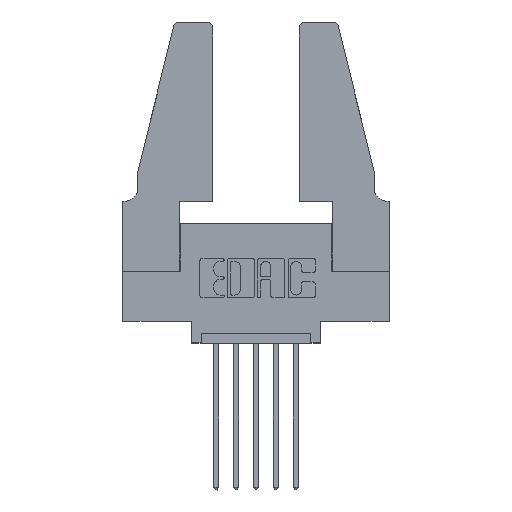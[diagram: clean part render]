
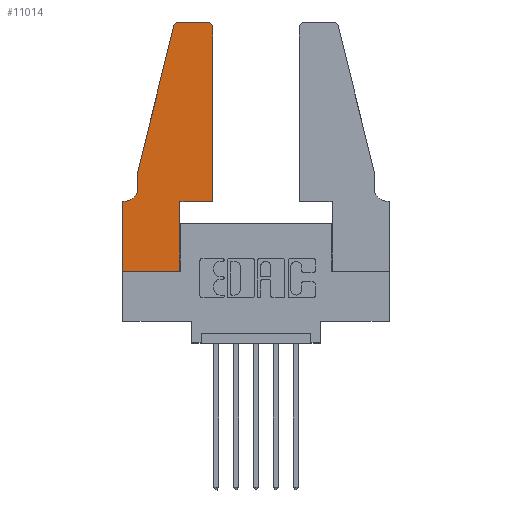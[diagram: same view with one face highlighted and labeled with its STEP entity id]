
A CAD part, top view. The second image highlights one B-rep face of the part: STEP entity #11014.
In plain terms, the highlighted planar face has unit normal (0, 0, 1).
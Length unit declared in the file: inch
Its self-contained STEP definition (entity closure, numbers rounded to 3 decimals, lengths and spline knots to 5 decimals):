
#429 = VERTEX_POINT ( 'NONE', #3707 ) ;
#541 = VECTOR ( 'NONE', #5327, 39.37008 ) ;
#584 = CARTESIAN_POINT ( 'NONE',  ( 0.4205, 1.25, 0.37 ) ) ;
#663 = CARTESIAN_POINT ( 'NONE',  ( 0., 0., 0.37 ) ) ;
#728 = CARTESIAN_POINT ( 'NONE',  ( 0.4505, 0.35, 0.37 ) ) ;
#730 = CIRCLE ( 'NONE', #3010, 0.03 ) ;
#745 = DIRECTION ( 'NONE',  ( -1., 0., 0. ) ) ;
#778 = CARTESIAN_POINT ( 'NONE',  ( 0.2865, 0.35, 0.37 ) ) ;
#1076 = ORIENTED_EDGE ( 'NONE', *, *, #3592, .T. ) ;
#1146 = LINE ( 'NONE', #728, #5699 ) ;
#1365 = DIRECTION ( 'NONE',  ( 1., 0., 0. ) ) ;
#1618 = DIRECTION ( 'NONE',  ( 0., 1., 0. ) ) ;
#1673 = DIRECTION ( 'NONE',  ( 0., 1., 0. ) ) ;
#1690 = CARTESIAN_POINT ( 'NONE',  ( 0.2865, 0., 0.37 ) ) ;
#1817 = VERTEX_POINT ( 'NONE', #10746 ) ;
#1918 = DIRECTION ( 'NONE',  ( -1., 0., 0. ) ) ;
#1926 = AXIS2_PLACEMENT_3D ( 'NONE', #5299, #6277, #3754 ) ;
#1953 = EDGE_CURVE ( 'NONE', #7931, #5678, #6716, .T. ) ;
#2191 = DIRECTION ( 'NONE',  ( -0.239, -0.971, 0. ) ) ;
#2199 = VERTEX_POINT ( 'NONE', #4493 ) ;
#2353 = VECTOR ( 'NONE', #1918, 39.37008 ) ;
#2553 = VECTOR ( 'NONE', #1365, 39.37008 ) ;
#2672 = EDGE_CURVE ( 'NONE', #7817, #1817, #7754, .T. ) ;
#2702 = EDGE_CURVE ( 'NONE', #5678, #7817, #6562, .T. ) ;
#2801 = CARTESIAN_POINT ( 'NONE',  ( 0., 0.35, 0.37 ) ) ;
#2839 = DIRECTION ( 'NONE',  ( 1., 0., 0. ) ) ;
#3010 = AXIS2_PLACEMENT_3D ( 'NONE', #9681, #10557, #8020 ) ;
#3168 = CARTESIAN_POINT ( 'NONE',  ( 0.0755, 0.5, 0.37 ) ) ;
#3229 = EDGE_CURVE ( 'NONE', #5174, #7931, #8313, .T. ) ;
#3278 = EDGE_CURVE ( 'NONE', #8522, #9363, #4676, .T. ) ;
#3303 = ORIENTED_EDGE ( 'NONE', *, *, #2702, .T. ) ;
#3383 = DIRECTION ( 'NONE',  ( 0., 0., -1. ) ) ;
#3541 = ORIENTED_EDGE ( 'NONE', *, *, #10497, .T. ) ;
#3592 = EDGE_CURVE ( 'NONE', #4419, #7984, #6683, .T. ) ;
#3603 = VECTOR ( 'NONE', #8098, 39.37008 ) ;
#3707 = CARTESIAN_POINT ( 'NONE',  ( 0.0755, 0.42, 0.37 ) ) ;
#3754 = DIRECTION ( 'NONE',  ( 1., 0., 0. ) ) ;
#3894 = DIRECTION ( 'NONE',  ( -1., 0., 0. ) ) ;
#4136 = CARTESIAN_POINT ( 'NONE',  ( 0., 0.35, 0.37 ) ) ;
#4389 = CIRCLE ( 'NONE', #1926, 0.03 ) ;
#4419 = VERTEX_POINT ( 'NONE', #4843 ) ;
#4493 = CARTESIAN_POINT ( 'NONE',  ( 0.0055, 0.35, 0.37 ) ) ;
#4636 = ORIENTED_EDGE ( 'NONE', *, *, #6787, .T. ) ;
#4676 = LINE ( 'NONE', #8047, #9889 ) ;
#4743 = VERTEX_POINT ( 'NONE', #5512 ) ;
#4843 = CARTESIAN_POINT ( 'NONE',  ( 0.25487, 1.22718, 0.37 ) ) ;
#4996 = CARTESIAN_POINT ( 'NONE',  ( 0., 0., 0.37 ) ) ;
#5074 = CARTESIAN_POINT ( 'NONE',  ( 0.0055, 0.42, 0.37 ) ) ;
#5125 = EDGE_CURVE ( 'NONE', #429, #2199, #5153, .T. ) ;
#5153 = CIRCLE ( 'NONE', #5465, 0.07 ) ;
#5174 = VERTEX_POINT ( 'NONE', #4136 ) ;
#5245 = EDGE_CURVE ( 'NONE', #1817, #4743, #1146, .T. ) ;
#5299 = CARTESIAN_POINT ( 'NONE',  ( 0.284, 1.22, 0.37 ) ) ;
#5319 = PLANE ( 'NONE',  #10430 ) ;
#5327 = DIRECTION ( 'NONE',  ( 0., -1., 0. ) ) ;
#5395 = ORIENTED_EDGE ( 'NONE', *, *, #1953, .T. ) ;
#5465 = AXIS2_PLACEMENT_3D ( 'NONE', #5074, #3383, #745 ) ;
#5492 = CARTESIAN_POINT ( 'NONE',  ( 0., 0., 0.37 ) ) ;
#5512 = CARTESIAN_POINT ( 'NONE',  ( 0.4505, 1.22, 0.37 ) ) ;
#5522 = EDGE_LOOP ( 'NONE', ( #10660, #10334, #1076, #4636, #9671, #3541, #5785, #5395, #3303, #7580, #6236, #7223 ) ) ;
#5678 = VERTEX_POINT ( 'NONE', #1690 ) ;
#5699 = VECTOR ( 'NONE', #1618, 39.37008 ) ;
#5785 = ORIENTED_EDGE ( 'NONE', *, *, #3229, .T. ) ;
#6120 = VECTOR ( 'NONE', #2191, 39.37008 ) ;
#6159 = CARTESIAN_POINT ( 'NONE',  ( 0.0755, 0.5, 0.37 ) ) ;
#6236 = ORIENTED_EDGE ( 'NONE', *, *, #5245, .T. ) ;
#6277 = DIRECTION ( 'NONE',  ( 0., 0., 1. ) ) ;
#6562 = LINE ( 'NONE', #778, #8584 ) ;
#6683 = LINE ( 'NONE', #7224, #6120 ) ;
#6716 = LINE ( 'NONE', #663, #9124 ) ;
#6787 = EDGE_CURVE ( 'NONE', #7984, #429, #9113, .T. ) ;
#6819 = CARTESIAN_POINT ( 'NONE',  ( 0.4505, 0.35, 0.37 ) ) ;
#7028 = CARTESIAN_POINT ( 'NONE',  ( 0.0755, 0.35, 0.37 ) ) ;
#7223 = ORIENTED_EDGE ( 'NONE', *, *, #10591, .T. ) ;
#7224 = CARTESIAN_POINT ( 'NONE',  ( 0.0755, 0.5, 0.37 ) ) ;
#7580 = ORIENTED_EDGE ( 'NONE', *, *, #2672, .T. ) ;
#7754 = LINE ( 'NONE', #6819, #2553 ) ;
#7817 = VERTEX_POINT ( 'NONE', #10988 ) ;
#7931 = VERTEX_POINT ( 'NONE', #4996 ) ;
#7984 = VERTEX_POINT ( 'NONE', #3168 ) ;
#8020 = DIRECTION ( 'NONE',  ( 1., 0., 0. ) ) ;
#8047 = CARTESIAN_POINT ( 'NONE',  ( 0.2605, 1.25, 0.37 ) ) ;
#8098 = DIRECTION ( 'NONE',  ( 0., -1., 0. ) ) ;
#8313 = LINE ( 'NONE', #5492, #3603 ) ;
#8522 = VERTEX_POINT ( 'NONE', #584 ) ;
#8584 = VECTOR ( 'NONE', #1673, 39.37008 ) ;
#8641 = LINE ( 'NONE', #7028, #2353 ) ;
#8749 = CARTESIAN_POINT ( 'NONE',  ( 0.284, 1.25, 0.37 ) ) ;
#8787 = DIRECTION ( 'NONE',  ( 0., 0., 1. ) ) ;
#9051 = EDGE_CURVE ( 'NONE', #9363, #4419, #4389, .T. ) ;
#9113 = LINE ( 'NONE', #6159, #541 ) ;
#9124 = VECTOR ( 'NONE', #9132, 39.37008 ) ;
#9132 = DIRECTION ( 'NONE',  ( 1., 0., 0. ) ) ;
#9363 = VERTEX_POINT ( 'NONE', #8749 ) ;
#9671 = ORIENTED_EDGE ( 'NONE', *, *, #5125, .T. ) ;
#9681 = CARTESIAN_POINT ( 'NONE',  ( 0.4205, 1.22, 0.37 ) ) ;
#9889 = VECTOR ( 'NONE', #3894, 39.37008 ) ;
#9964 = FACE_OUTER_BOUND ( 'NONE', #5522, .T. ) ;
#10334 = ORIENTED_EDGE ( 'NONE', *, *, #9051, .T. ) ;
#10430 = AXIS2_PLACEMENT_3D ( 'NONE', #2801, #8787, #2839 ) ;
#10497 = EDGE_CURVE ( 'NONE', #2199, #5174, #8641, .T. ) ;
#10557 = DIRECTION ( 'NONE',  ( 0., 0., 1. ) ) ;
#10591 = EDGE_CURVE ( 'NONE', #4743, #8522, #730, .T. ) ;
#10660 = ORIENTED_EDGE ( 'NONE', *, *, #3278, .T. ) ;
#10746 = CARTESIAN_POINT ( 'NONE',  ( 0.4505, 0.35, 0.37 ) ) ;
#10988 = CARTESIAN_POINT ( 'NONE',  ( 0.2865, 0.35, 0.37 ) ) ;
#11014 = ADVANCED_FACE ( 'NONE', ( #9964 ), #5319, .T. ) ;
